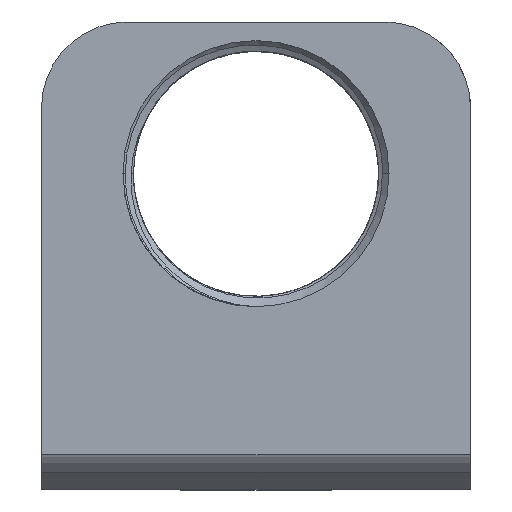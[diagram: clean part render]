
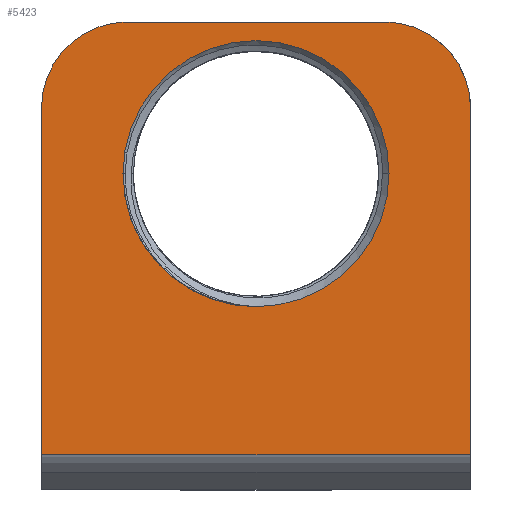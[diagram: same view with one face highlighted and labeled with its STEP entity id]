
A CAD part, top view. The second image highlights one B-rep face of the part: STEP entity #5423.
In plain terms, the highlighted planar face has unit normal (0, 0, 1).
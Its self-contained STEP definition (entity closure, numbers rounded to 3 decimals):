
#926 = AXIS2_PLACEMENT_3D ( 'NONE', #35521, #14733, #39018 ) ;
#1530 = CARTESIAN_POINT ( 'NONE',  ( 15.506, 0., 13.224 ) ) ;
#1609 = EDGE_CURVE ( 'NONE', #44860, #2925, #36994, .T. ) ;
#2167 = CIRCLE ( 'NONE', #926, 10. ) ;
#2925 = VERTEX_POINT ( 'NONE', #37108 ) ;
#3060 = CARTESIAN_POINT ( 'NONE',  ( 0., 17.678, 13.224 ) ) ;
#3383 = VERTEX_POINT ( 'NONE', #22711 ) ;
#3526 = CARTESIAN_POINT ( 'NONE',  ( 0., 0., 13.224 ) ) ;
#4177 = ORIENTED_EDGE ( 'NONE', *, *, #26373, .T. ) ;
#4290 = PLANE ( 'NONE',  #17247 ) ;
#4340 = CARTESIAN_POINT ( 'NONE',  ( -25., -32.779, 13.224 ) ) ;
#4396 = DIRECTION ( 'NONE',  ( 0., 0., -1. ) ) ;
#5043 = EDGE_CURVE ( 'NONE', #23124, #8799, #2167, .T. ) ;
#5423 = ADVANCED_FACE ( 'NONE', ( #36952, #12531 ), #4290, .T. ) ;
#6575 = DIRECTION ( 'NONE',  ( -1., 0., 0. ) ) ;
#7041 = DIRECTION ( 'NONE',  ( -1., 0., 0. ) ) ;
#7684 = LINE ( 'NONE', #4340, #43530 ) ;
#7797 = CARTESIAN_POINT ( 'NONE',  ( 0., 0., 13.224 ) ) ;
#7847 = DIRECTION ( 'NONE',  ( 1., 0., 0. ) ) ;
#8132 = LINE ( 'NONE', #3060, #34767 ) ;
#8510 = CARTESIAN_POINT ( 'NONE',  ( -15.506, 0., 13.224 ) ) ;
#8799 = VERTEX_POINT ( 'NONE', #37266 ) ;
#9352 = VERTEX_POINT ( 'NONE', #20110 ) ;
#10651 = ORIENTED_EDGE ( 'NONE', *, *, #14767, .T. ) ;
#11151 = ORIENTED_EDGE ( 'NONE', *, *, #5043, .T. ) ;
#12531 = FACE_OUTER_BOUND ( 'NONE', #39938, .T. ) ;
#13047 = LINE ( 'NONE', #14166, #21173 ) ;
#13761 = DIRECTION ( 'NONE',  ( 0., 0., -1. ) ) ;
#14166 = CARTESIAN_POINT ( 'NONE',  ( 25., 0., 13.224 ) ) ;
#14381 = CIRCLE ( 'NONE', #44632, 15.506 ) ;
#14531 = DIRECTION ( 'NONE',  ( 0., 0., 1. ) ) ;
#14733 = DIRECTION ( 'NONE',  ( 0., 0., 1. ) ) ;
#14767 = EDGE_CURVE ( 'NONE', #3383, #20901, #14381, .T. ) ;
#15327 = CARTESIAN_POINT ( 'NONE',  ( -25., -32.779, 13.224 ) ) ;
#16216 = EDGE_CURVE ( 'NONE', #2925, #43030, #32263, .T. ) ;
#17247 = AXIS2_PLACEMENT_3D ( 'NONE', #7797, #18270, #42557 ) ;
#17904 = CIRCLE ( 'NONE', #27178, 15.506 ) ;
#18270 = DIRECTION ( 'NONE',  ( 0., 0., 1. ) ) ;
#18677 = EDGE_CURVE ( 'NONE', #34072, #3383, #37682, .T. ) ;
#18742 = AXIS2_PLACEMENT_3D ( 'NONE', #3526, #27840, #7041 ) ;
#19189 = AXIS2_PLACEMENT_3D ( 'NONE', #35314, #14531, #38805 ) ;
#20110 = CARTESIAN_POINT ( 'NONE',  ( 25., -32.779, 13.224 ) ) ;
#20901 = VERTEX_POINT ( 'NONE', #8510 ) ;
#21173 = VECTOR ( 'NONE', #27977, 1000. ) ;
#22711 = CARTESIAN_POINT ( 'NONE',  ( -0.03, -15.506, 13.224 ) ) ;
#23045 = CARTESIAN_POINT ( 'NONE',  ( -25., 0., 13.224 ) ) ;
#23124 = VERTEX_POINT ( 'NONE', #35049 ) ;
#24084 = ORIENTED_EDGE ( 'NONE', *, *, #1609, .T. ) ;
#25220 = CARTESIAN_POINT ( 'NONE',  ( 0., 0., 13.224 ) ) ;
#25353 = EDGE_LOOP ( 'NONE', ( #10651, #33172, #36196 ) ) ;
#26373 = EDGE_CURVE ( 'NONE', #43030, #9352, #7684, .T. ) ;
#26543 = DIRECTION ( 'NONE',  ( 0., -1., 0. ) ) ;
#27178 = AXIS2_PLACEMENT_3D ( 'NONE', #25220, #4396, #28705 ) ;
#27840 = DIRECTION ( 'NONE',  ( 0., 0., -1. ) ) ;
#27977 = DIRECTION ( 'NONE',  ( 0., 1., 0. ) ) ;
#28705 = DIRECTION ( 'NONE',  ( -1., 0., 0. ) ) ;
#28777 = EDGE_CURVE ( 'NONE', #8799, #44860, #8132, .T. ) ;
#29561 = EDGE_CURVE ( 'NONE', #9352, #23124, #13047, .T. ) ;
#30169 = EDGE_CURVE ( 'NONE', #20901, #34072, #17904, .T. ) ;
#31965 = CARTESIAN_POINT ( 'NONE',  ( -15., 17.678, 13.224 ) ) ;
#32263 = LINE ( 'NONE', #23045, #35538 ) ;
#33172 = ORIENTED_EDGE ( 'NONE', *, *, #30169, .T. ) ;
#34072 = VERTEX_POINT ( 'NONE', #1530 ) ;
#34551 = CARTESIAN_POINT ( 'NONE',  ( 0., 0., 13.224 ) ) ;
#34767 = VECTOR ( 'NONE', #6575, 1000. ) ;
#35049 = CARTESIAN_POINT ( 'NONE',  ( 25., 7.678, 13.224 ) ) ;
#35314 = CARTESIAN_POINT ( 'NONE',  ( -15., 7.678, 13.224 ) ) ;
#35415 = ORIENTED_EDGE ( 'NONE', *, *, #16216, .T. ) ;
#35521 = CARTESIAN_POINT ( 'NONE',  ( 15., 7.678, 13.224 ) ) ;
#35538 = VECTOR ( 'NONE', #26543, 1000. ) ;
#36196 = ORIENTED_EDGE ( 'NONE', *, *, #18677, .T. ) ;
#36952 = FACE_BOUND ( 'NONE', #25353, .T. ) ;
#36994 = CIRCLE ( 'NONE', #19189, 10. ) ;
#37108 = CARTESIAN_POINT ( 'NONE',  ( -25., 7.678, 13.224 ) ) ;
#37266 = CARTESIAN_POINT ( 'NONE',  ( 15., 17.678, 13.224 ) ) ;
#37682 = CIRCLE ( 'NONE', #18742, 15.506 ) ;
#38043 = DIRECTION ( 'NONE',  ( -1., 0., 0. ) ) ;
#38805 = DIRECTION ( 'NONE',  ( 1., 0., 0. ) ) ;
#39018 = DIRECTION ( 'NONE',  ( 1., 0., 0. ) ) ;
#39938 = EDGE_LOOP ( 'NONE', ( #4177, #40296, #11151, #44830, #24084, #35415 ) ) ;
#40296 = ORIENTED_EDGE ( 'NONE', *, *, #29561, .T. ) ;
#42557 = DIRECTION ( 'NONE',  ( 1., 0., 0. ) ) ;
#43030 = VERTEX_POINT ( 'NONE', #15327 ) ;
#43530 = VECTOR ( 'NONE', #7847, 1000. ) ;
#44632 = AXIS2_PLACEMENT_3D ( 'NONE', #34551, #13761, #38043 ) ;
#44830 = ORIENTED_EDGE ( 'NONE', *, *, #28777, .T. ) ;
#44860 = VERTEX_POINT ( 'NONE', #31965 ) ;
